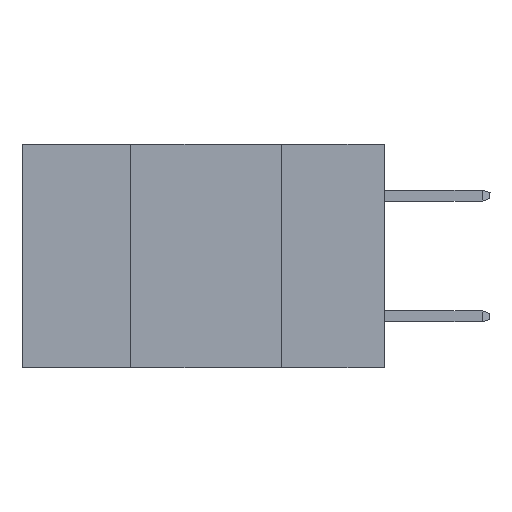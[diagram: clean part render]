
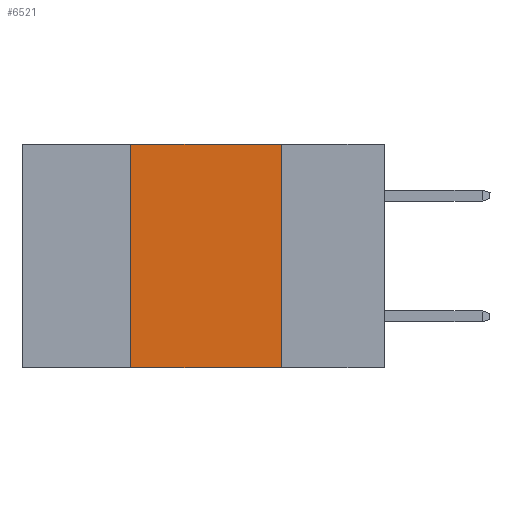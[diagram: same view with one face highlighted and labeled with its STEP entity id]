
A CAD part, left-side view. The second image highlights one B-rep face of the part: STEP entity #6521.
In plain terms, the highlighted planar face has unit normal (-1, 0, 0).
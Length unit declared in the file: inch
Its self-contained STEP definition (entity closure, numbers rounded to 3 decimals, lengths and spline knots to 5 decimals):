
#740 = EDGE_CURVE ( 'NONE', #22999, #16578, #4152, .T. ) ;
#963 = CARTESIAN_POINT ( 'NONE',  ( 0., 0.6, 0. ) ) ;
#1440 = VECTOR ( 'NONE', #19714, 39.37008 ) ;
#1589 = CARTESIAN_POINT ( 'NONE',  ( 0., 0.42, 0. ) ) ;
#2370 = EDGE_LOOP ( 'NONE', ( #19236, #3210, #4537, #11070 ) ) ;
#2742 = VECTOR ( 'NONE', #18217, 39.37008 ) ;
#3210 = ORIENTED_EDGE ( 'NONE', *, *, #11224, .F. ) ;
#4152 = LINE ( 'NONE', #24018, #8295 ) ;
#4537 = ORIENTED_EDGE ( 'NONE', *, *, #740, .F. ) ;
#4783 = CARTESIAN_POINT ( 'NONE',  ( 0., 0.42, -0.37 ) ) ;
#6151 = LINE ( 'NONE', #963, #1440 ) ;
#6521 = ADVANCED_FACE ( 'NONE', ( #7841 ), #9654, .F. ) ;
#7221 = CARTESIAN_POINT ( 'NONE',  ( 0., 0.17, 0. ) ) ;
#7841 = FACE_OUTER_BOUND ( 'NONE', #2370, .T. ) ;
#8295 = VECTOR ( 'NONE', #18681, 39.37008 ) ;
#9654 = PLANE ( 'NONE',  #9741 ) ;
#9741 = AXIS2_PLACEMENT_3D ( 'NONE', #20997, #11575, #9804 ) ;
#9804 = DIRECTION ( 'NONE',  ( 0., 0., -1. ) ) ;
#10189 = LINE ( 'NONE', #7221, #21303 ) ;
#10491 = VERTEX_POINT ( 'NONE', #19512 ) ;
#11070 = ORIENTED_EDGE ( 'NONE', *, *, #23187, .T. ) ;
#11224 = EDGE_CURVE ( 'NONE', #16578, #10491, #6151, .T. ) ;
#11575 = DIRECTION ( 'NONE',  ( 1., 0., 0. ) ) ;
#11840 = EDGE_CURVE ( 'NONE', #10491, #17286, #10189, .T. ) ;
#16578 = VERTEX_POINT ( 'NONE', #1589 ) ;
#16609 = CARTESIAN_POINT ( 'NONE',  ( 0., 0.6, -0.37 ) ) ;
#17286 = VERTEX_POINT ( 'NONE', #20881 ) ;
#18217 = DIRECTION ( 'NONE',  ( 0., -1., 0. ) ) ;
#18280 = LINE ( 'NONE', #16609, #2742 ) ;
#18681 = DIRECTION ( 'NONE',  ( 0., 0., 1. ) ) ;
#19236 = ORIENTED_EDGE ( 'NONE', *, *, #11840, .F. ) ;
#19512 = CARTESIAN_POINT ( 'NONE',  ( 0., 0.17, 0. ) ) ;
#19714 = DIRECTION ( 'NONE',  ( 0., -1., 0. ) ) ;
#20881 = CARTESIAN_POINT ( 'NONE',  ( 0., 0.17, -0.37 ) ) ;
#20997 = CARTESIAN_POINT ( 'NONE',  ( 0., 0.6, 0. ) ) ;
#21303 = VECTOR ( 'NONE', #22193, 39.37008 ) ;
#22193 = DIRECTION ( 'NONE',  ( 0., 0., -1. ) ) ;
#22999 = VERTEX_POINT ( 'NONE', #4783 ) ;
#23187 = EDGE_CURVE ( 'NONE', #22999, #17286, #18280, .T. ) ;
#24018 = CARTESIAN_POINT ( 'NONE',  ( 0., 0.42, 0. ) ) ;
